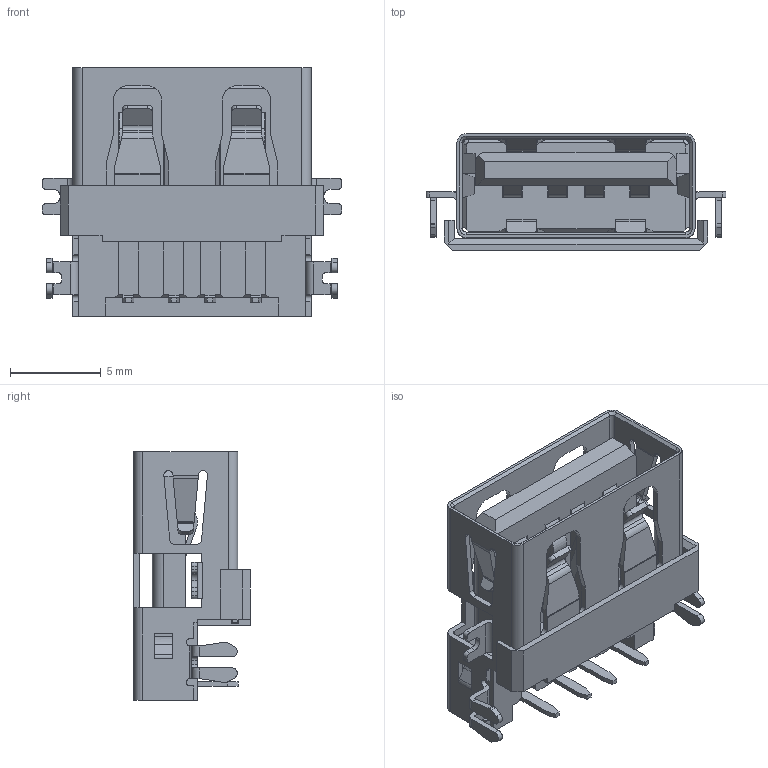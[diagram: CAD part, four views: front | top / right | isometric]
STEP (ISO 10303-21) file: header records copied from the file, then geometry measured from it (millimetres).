
FILE_DESCRIPTION (( 'STEP AP214' ), '1' );
FILE_NAME ('690G104-159-241.STEP', '2021-01-14T13:47:26', ( '' ), ( '' ), 'SwSTEP 2.0', 'SolidWorks 2020', '' );
FILE_SCHEMA (( 'AUTOMOTIVE_DESIGN' ));
Length unit declared in the file: millimetre
Products named in the file (4): Shell 690G104-X59-24X; Contacts 690G104-X59-24X; 690G104-159-241; Insulator 690G104-X59-24X_Black
Assembly tree (3 placements, depth 2):
  690G104-159-241
    Insulator 690G104-X59-24X_Black
    Contacts 690G104-X59-24X
    Shell 690G104-X59-24X
Bounding box: 16.5 x 6.42 x 13.7 mm (x, y, z)
Volume: 416.7 mm3; surface area: 1719 mm2
Topology: 6 solids, 6 shells, 800 faces, 2293 edges, 1491 vertices
Faces by surface type: plane 585, cylinder 185, bspline 24, cone 6
Entity records: 27212 total; most frequent: CARTESIAN_POINT 6348, ORIENTED_EDGE 4586, DIRECTION 3913, EDGE_CURVE 2293, LINE 1829, VECTOR 1829, VERTEX_POINT 1491, AXIS2_PLACEMENT_3D 1042
